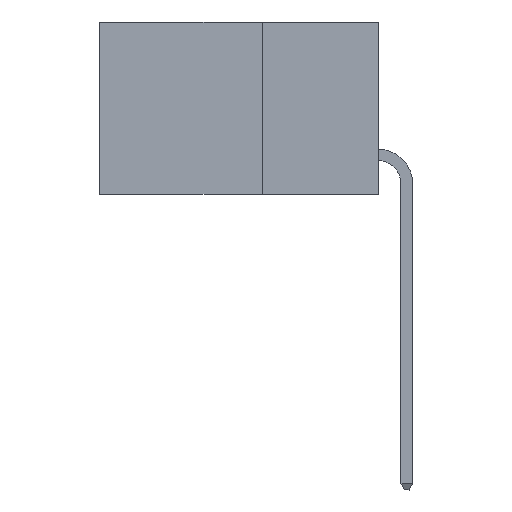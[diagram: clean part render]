
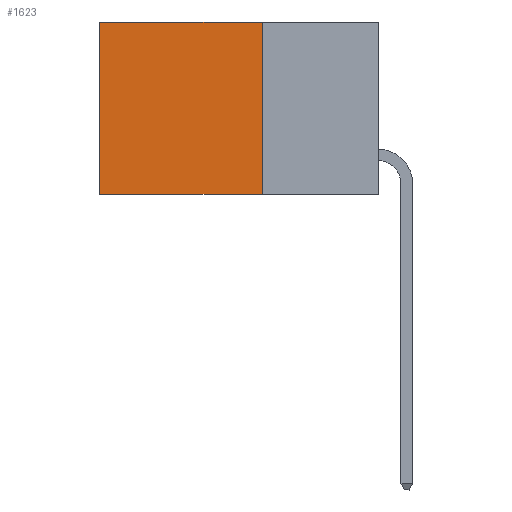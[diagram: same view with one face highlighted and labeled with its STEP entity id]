
A CAD part, left-side view. The second image highlights one B-rep face of the part: STEP entity #1623.
In plain terms, the highlighted planar face has unit normal (-1, 0, 0).
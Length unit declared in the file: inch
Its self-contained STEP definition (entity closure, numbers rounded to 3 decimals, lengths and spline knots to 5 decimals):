
#508 = DIRECTION ( 'NONE',  ( 0., 0., -1. ) ) ;
#1310 = DIRECTION ( 'NONE',  ( 0., 0., -1. ) ) ;
#1623 = ADVANCED_FACE ( 'NONE', ( #20677 ), #24012, .F. ) ;
#2310 = ORIENTED_EDGE ( 'NONE', *, *, #16877, .T. ) ;
#2649 = DIRECTION ( 'NONE',  ( 0., 0., -1. ) ) ;
#2742 = CARTESIAN_POINT ( 'NONE',  ( 0.298, 0.6, 0. ) ) ;
#3032 = EDGE_CURVE ( 'NONE', #10592, #5630, #10981, .T. ) ;
#4423 = CARTESIAN_POINT ( 'NONE',  ( 0.298, 0.6, -0.37 ) ) ;
#5630 = VERTEX_POINT ( 'NONE', #6430 ) ;
#5676 = DIRECTION ( 'NONE',  ( 0., 1., 0. ) ) ;
#6430 = CARTESIAN_POINT ( 'NONE',  ( 0.298, 0.25, -0.37 ) ) ;
#7121 = CARTESIAN_POINT ( 'NONE',  ( 0.298, 0.25, 0. ) ) ;
#9443 = EDGE_LOOP ( 'NONE', ( #11591, #14101, #24959, #2310 ) ) ;
#9724 = CARTESIAN_POINT ( 'NONE',  ( 0.298, 0.6, 0. ) ) ;
#10035 = DIRECTION ( 'NONE',  ( 1., 0., 0. ) ) ;
#10592 = VERTEX_POINT ( 'NONE', #23990 ) ;
#10981 = LINE ( 'NONE', #7121, #14728 ) ;
#11591 = ORIENTED_EDGE ( 'NONE', *, *, #24605, .T. ) ;
#12001 = VECTOR ( 'NONE', #14856, 39.37008 ) ;
#14036 = CARTESIAN_POINT ( 'NONE',  ( 0.298, 0.25, 0. ) ) ;
#14101 = ORIENTED_EDGE ( 'NONE', *, *, #24295, .F. ) ;
#14197 = LINE ( 'NONE', #14770, #12001 ) ;
#14541 = LINE ( 'NONE', #25586, #17929 ) ;
#14728 = VECTOR ( 'NONE', #1310, 39.37008 ) ;
#14770 = CARTESIAN_POINT ( 'NONE',  ( 0.298, 0.25, -0.37 ) ) ;
#14856 = DIRECTION ( 'NONE',  ( 0., 1., 0. ) ) ;
#16877 = EDGE_CURVE ( 'NONE', #10592, #21638, #14541, .T. ) ;
#17929 = VECTOR ( 'NONE', #5676, 39.37008 ) ;
#20677 = FACE_OUTER_BOUND ( 'NONE', #9443, .T. ) ;
#21638 = VERTEX_POINT ( 'NONE', #9724 ) ;
#22195 = LINE ( 'NONE', #2742, #23445 ) ;
#23445 = VECTOR ( 'NONE', #508, 39.37008 ) ;
#23990 = CARTESIAN_POINT ( 'NONE',  ( 0.298, 0.25, 0. ) ) ;
#24012 = PLANE ( 'NONE',  #24155 ) ;
#24155 = AXIS2_PLACEMENT_3D ( 'NONE', #14036, #10035, #2649 ) ;
#24295 = EDGE_CURVE ( 'NONE', #5630, #24688, #14197, .T. ) ;
#24605 = EDGE_CURVE ( 'NONE', #21638, #24688, #22195, .T. ) ;
#24688 = VERTEX_POINT ( 'NONE', #4423 ) ;
#24959 = ORIENTED_EDGE ( 'NONE', *, *, #3032, .F. ) ;
#25586 = CARTESIAN_POINT ( 'NONE',  ( 0.298, 0.25, 0. ) ) ;
